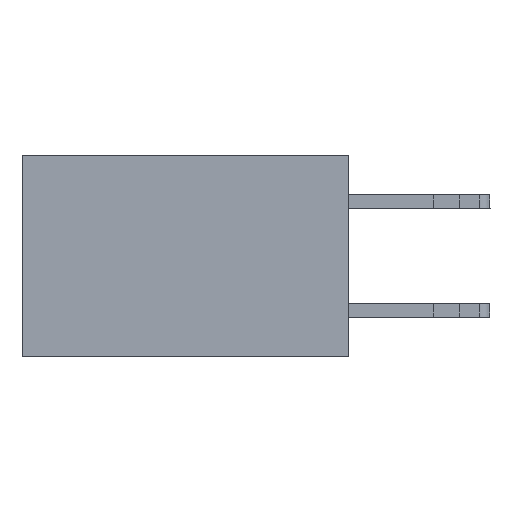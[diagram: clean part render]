
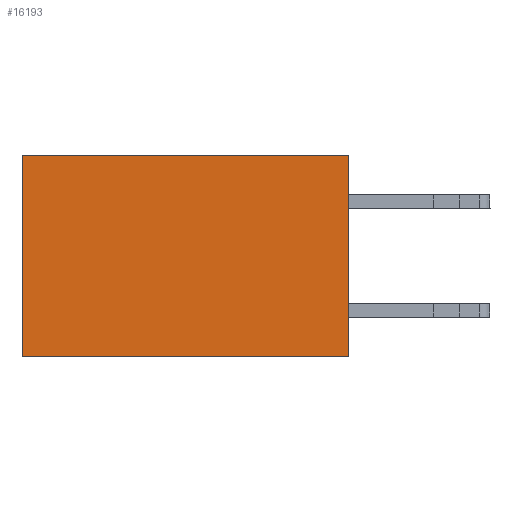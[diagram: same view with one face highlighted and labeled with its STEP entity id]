
A CAD part, left-side view. The second image highlights one B-rep face of the part: STEP entity #16193.
In plain terms, the highlighted planar face has unit normal (-1, 0, 0).
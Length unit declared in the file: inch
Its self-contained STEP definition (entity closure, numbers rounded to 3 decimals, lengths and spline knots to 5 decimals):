
#361 = PLANE ( 'NONE',  #9510 ) ;
#824 = VERTEX_POINT ( 'NONE', #5323 ) ;
#2055 = VERTEX_POINT ( 'NONE', #16423 ) ;
#2451 = EDGE_CURVE ( 'NONE', #17755, #16319, #3604, .T. ) ;
#2558 = VECTOR ( 'NONE', #10502, 39.37008 ) ;
#2574 = VECTOR ( 'NONE', #5124, 39.37008 ) ;
#2950 = VECTOR ( 'NONE', #6299, 39.37008 ) ;
#3604 = LINE ( 'NONE', #8057, #2558 ) ;
#5124 = DIRECTION ( 'NONE',  ( 0., 0., -1. ) ) ;
#5323 = CARTESIAN_POINT ( 'NONE',  ( 0.2615, 0.6, -0.37 ) ) ;
#6233 = EDGE_CURVE ( 'NONE', #17755, #2055, #10122, .T. ) ;
#6299 = DIRECTION ( 'NONE',  ( 0., 1., 0. ) ) ;
#6674 = EDGE_LOOP ( 'NONE', ( #11262, #10570, #7523, #7770 ) ) ;
#6736 = CARTESIAN_POINT ( 'NONE',  ( 0.2615, 0., 0. ) ) ;
#7153 = EDGE_CURVE ( 'NONE', #2055, #824, #14467, .T. ) ;
#7188 = FACE_OUTER_BOUND ( 'NONE', #6674, .T. ) ;
#7523 = ORIENTED_EDGE ( 'NONE', *, *, #6233, .F. ) ;
#7561 = EDGE_CURVE ( 'NONE', #16319, #824, #7778, .T. ) ;
#7648 = CARTESIAN_POINT ( 'NONE',  ( 0.2615, 0.6, 0. ) ) ;
#7770 = ORIENTED_EDGE ( 'NONE', *, *, #2451, .T. ) ;
#7778 = LINE ( 'NONE', #11840, #2574 ) ;
#8057 = CARTESIAN_POINT ( 'NONE',  ( 0.2615, 0., 0. ) ) ;
#8492 = DIRECTION ( 'NONE',  ( 0., 0., -1. ) ) ;
#9510 = AXIS2_PLACEMENT_3D ( 'NONE', #15623, #12705, #10003 ) ;
#10003 = DIRECTION ( 'NONE',  ( 0., 0., -1. ) ) ;
#10122 = LINE ( 'NONE', #11400, #15959 ) ;
#10502 = DIRECTION ( 'NONE',  ( 0., 1., 0. ) ) ;
#10570 = ORIENTED_EDGE ( 'NONE', *, *, #7153, .F. ) ;
#11262 = ORIENTED_EDGE ( 'NONE', *, *, #7561, .T. ) ;
#11400 = CARTESIAN_POINT ( 'NONE',  ( 0.2615, 0., -0.37 ) ) ;
#11840 = CARTESIAN_POINT ( 'NONE',  ( 0.2615, 0.6, -0.37 ) ) ;
#11914 = CARTESIAN_POINT ( 'NONE',  ( 0.2615, 0., -0.37 ) ) ;
#12705 = DIRECTION ( 'NONE',  ( 1., 0., 0. ) ) ;
#14467 = LINE ( 'NONE', #11914, #2950 ) ;
#15623 = CARTESIAN_POINT ( 'NONE',  ( 0.2615, 0., -0.37 ) ) ;
#15959 = VECTOR ( 'NONE', #8492, 39.37008 ) ;
#16193 = ADVANCED_FACE ( 'NONE', ( #7188 ), #361, .F. ) ;
#16319 = VERTEX_POINT ( 'NONE', #7648 ) ;
#16423 = CARTESIAN_POINT ( 'NONE',  ( 0.2615, 0., -0.37 ) ) ;
#17755 = VERTEX_POINT ( 'NONE', #6736 ) ;
